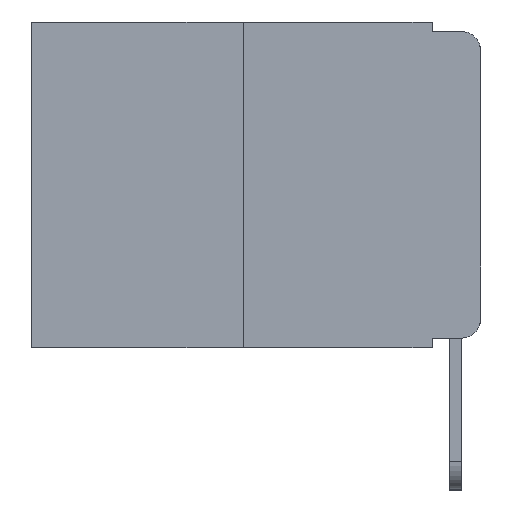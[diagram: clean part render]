
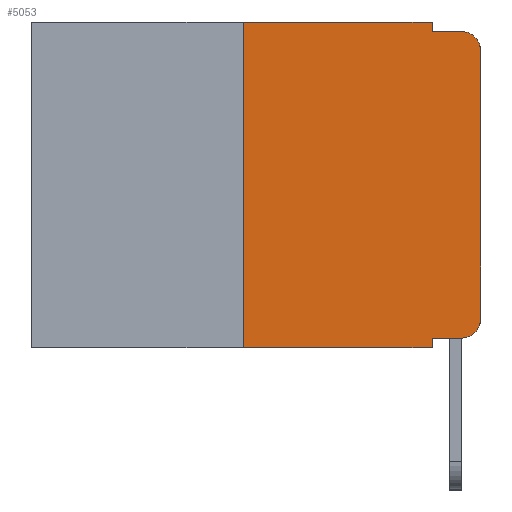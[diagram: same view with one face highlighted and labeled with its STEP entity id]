
A CAD part, left-side view. The second image highlights one B-rep face of the part: STEP entity #5053.
In plain terms, the highlighted planar face has unit normal (-1, 0, 0).
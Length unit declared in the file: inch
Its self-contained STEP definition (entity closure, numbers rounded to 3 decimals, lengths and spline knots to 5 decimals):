
#15 = CARTESIAN_POINT ( 'NONE',  ( 0., 0.051, 0. ) ) ;
#44 = CARTESIAN_POINT ( 'NONE',  ( 0., 0.473, 0. ) ) ;
#75 = CARTESIAN_POINT ( 'NONE',  ( 0., 0., -0.313 ) ) ;
#151 = ORIENTED_EDGE ( 'NONE', *, *, #8864, .F. ) ;
#792 = DIRECTION ( 'NONE',  ( 1., 0., 0. ) ) ;
#899 = LINE ( 'NONE', #6831, #10990 ) ;
#989 = EDGE_CURVE ( 'NONE', #1413, #6088, #6615, .T. ) ;
#1100 = VERTEX_POINT ( 'NONE', #75 ) ;
#1357 = LINE ( 'NONE', #15, #12115 ) ;
#1382 = CIRCLE ( 'NONE', #13444, 0.02 ) ;
#1402 = LINE ( 'NONE', #2084, #12153 ) ;
#1413 = VERTEX_POINT ( 'NONE', #8757 ) ;
#1432 = ORIENTED_EDGE ( 'NONE', *, *, #6324, .F. ) ;
#1491 = CARTESIAN_POINT ( 'NONE',  ( 0., 0.02, -0.313 ) ) ;
#1691 = VECTOR ( 'NONE', #3084, 39.37008 ) ;
#2036 = DIRECTION ( 'NONE',  ( 0., 0., -1. ) ) ;
#2084 = CARTESIAN_POINT ( 'NONE',  ( 0., 0.051, 0. ) ) ;
#2368 = CARTESIAN_POINT ( 'NONE',  ( 0., 0.051, -0.333 ) ) ;
#2591 = CARTESIAN_POINT ( 'NONE',  ( 0., 0.051, -0.333 ) ) ;
#2603 = ORIENTED_EDGE ( 'NONE', *, *, #11620, .T. ) ;
#2794 = EDGE_CURVE ( 'NONE', #1100, #7770, #6084, .T. ) ;
#2942 = CARTESIAN_POINT ( 'NONE',  ( 0., 0.051, -0.01 ) ) ;
#3084 = DIRECTION ( 'NONE',  ( 0., -1., 0. ) ) ;
#3243 = EDGE_CURVE ( 'NONE', #6088, #7685, #1402, .T. ) ;
#3689 = FACE_OUTER_BOUND ( 'NONE', #8586, .T. ) ;
#3717 = VECTOR ( 'NONE', #9342, 39.37008 ) ;
#3837 = EDGE_CURVE ( 'NONE', #6520, #12544, #13106, .T. ) ;
#4094 = LINE ( 'NONE', #2591, #5881 ) ;
#4596 = ORIENTED_EDGE ( 'NONE', *, *, #989, .F. ) ;
#4703 = DIRECTION ( 'NONE',  ( -1., 0., 0. ) ) ;
#4867 = ORIENTED_EDGE ( 'NONE', *, *, #7696, .F. ) ;
#5053 = ADVANCED_FACE ( 'NONE', ( #3689 ), #12409, .F. ) ;
#5241 = CARTESIAN_POINT ( 'NONE',  ( 0., 0.051, -0.343 ) ) ;
#5632 = DIRECTION ( 'NONE',  ( 0., 0., -1. ) ) ;
#5881 = VECTOR ( 'NONE', #9724, 39.37008 ) ;
#6084 = LINE ( 'NONE', #7835, #7548 ) ;
#6088 = VERTEX_POINT ( 'NONE', #12314 ) ;
#6113 = CARTESIAN_POINT ( 'NONE',  ( 0., 0.02, -0.03 ) ) ;
#6168 = ORIENTED_EDGE ( 'NONE', *, *, #7056, .T. ) ;
#6290 = ORIENTED_EDGE ( 'NONE', *, *, #12909, .T. ) ;
#6324 = EDGE_CURVE ( 'NONE', #6520, #1413, #899, .T. ) ;
#6520 = VERTEX_POINT ( 'NONE', #7940 ) ;
#6615 = LINE ( 'NONE', #44, #3717 ) ;
#6809 = ORIENTED_EDGE ( 'NONE', *, *, #2794, .T. ) ;
#6831 = CARTESIAN_POINT ( 'NONE',  ( 0., 0.25, 0. ) ) ;
#6887 = ORIENTED_EDGE ( 'NONE', *, *, #3837, .T. ) ;
#7056 = EDGE_CURVE ( 'NONE', #7770, #13068, #1382, .T. ) ;
#7058 = CARTESIAN_POINT ( 'NONE',  ( 0., 0.473, 0. ) ) ;
#7208 = VECTOR ( 'NONE', #7272, 39.37008 ) ;
#7272 = DIRECTION ( 'NONE',  ( 0., -1., 0. ) ) ;
#7548 = VECTOR ( 'NONE', #8797, 39.37008 ) ;
#7685 = VERTEX_POINT ( 'NONE', #2942 ) ;
#7696 = EDGE_CURVE ( 'NONE', #7685, #13068, #7871, .T. ) ;
#7770 = VERTEX_POINT ( 'NONE', #9397 ) ;
#7835 = CARTESIAN_POINT ( 'NONE',  ( 0., 0., 0. ) ) ;
#7871 = LINE ( 'NONE', #10253, #7208 ) ;
#7934 = DIRECTION ( 'NONE',  ( 0., 0., 1. ) ) ;
#7940 = CARTESIAN_POINT ( 'NONE',  ( 0., 0.25, -0.343 ) ) ;
#8169 = DIRECTION ( 'NONE',  ( 0., 0., -1. ) ) ;
#8520 = AXIS2_PLACEMENT_3D ( 'NONE', #7058, #792, #8169 ) ;
#8586 = EDGE_LOOP ( 'NONE', ( #6809, #6168, #4867, #12131, #4596, #1432, #6887, #151, #6290, #2603 ) ) ;
#8757 = CARTESIAN_POINT ( 'NONE',  ( 0., 0.25, 0. ) ) ;
#8797 = DIRECTION ( 'NONE',  ( 0., 0., 1. ) ) ;
#8864 = EDGE_CURVE ( 'NONE', #9021, #12544, #1357, .T. ) ;
#9021 = VERTEX_POINT ( 'NONE', #2368 ) ;
#9321 = DIRECTION ( 'NONE',  ( 0., 0., -1. ) ) ;
#9342 = DIRECTION ( 'NONE',  ( 0., -1., 0. ) ) ;
#9397 = CARTESIAN_POINT ( 'NONE',  ( 0., 0., -0.03 ) ) ;
#9724 = DIRECTION ( 'NONE',  ( 0., -1., 0. ) ) ;
#10183 = DIRECTION ( 'NONE',  ( 0., 0., -1. ) ) ;
#10224 = DIRECTION ( 'NONE',  ( -1., 0., 0. ) ) ;
#10253 = CARTESIAN_POINT ( 'NONE',  ( 0., 0.051, -0.01 ) ) ;
#10267 = CARTESIAN_POINT ( 'NONE',  ( 0., 0.02, -0.01 ) ) ;
#10350 = CARTESIAN_POINT ( 'NONE',  ( 0., 0.473, -0.343 ) ) ;
#10990 = VECTOR ( 'NONE', #7934, 39.37008 ) ;
#11620 = EDGE_CURVE ( 'NONE', #13367, #1100, #12795, .T. ) ;
#12019 = AXIS2_PLACEMENT_3D ( 'NONE', #1491, #4703, #5632 ) ;
#12115 = VECTOR ( 'NONE', #9321, 39.37008 ) ;
#12131 = ORIENTED_EDGE ( 'NONE', *, *, #3243, .F. ) ;
#12153 = VECTOR ( 'NONE', #2036, 39.37008 ) ;
#12254 = CARTESIAN_POINT ( 'NONE',  ( 0., 0.02, -0.333 ) ) ;
#12314 = CARTESIAN_POINT ( 'NONE',  ( 0., 0.051, 0. ) ) ;
#12409 = PLANE ( 'NONE',  #8520 ) ;
#12544 = VERTEX_POINT ( 'NONE', #5241 ) ;
#12795 = CIRCLE ( 'NONE', #12019, 0.02 ) ;
#12909 = EDGE_CURVE ( 'NONE', #9021, #13367, #4094, .T. ) ;
#13068 = VERTEX_POINT ( 'NONE', #10267 ) ;
#13106 = LINE ( 'NONE', #10350, #1691 ) ;
#13367 = VERTEX_POINT ( 'NONE', #12254 ) ;
#13444 = AXIS2_PLACEMENT_3D ( 'NONE', #6113, #10224, #10183 ) ;
